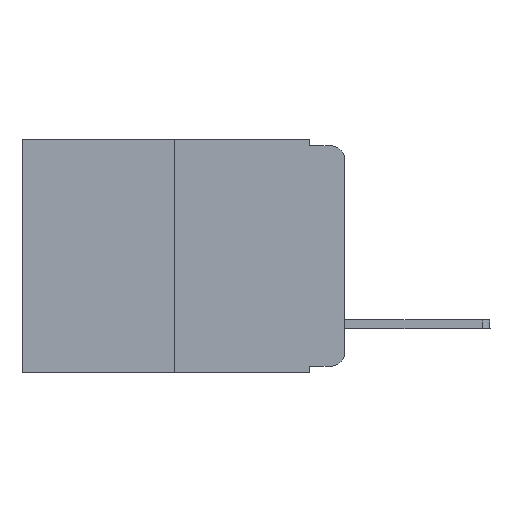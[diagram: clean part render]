
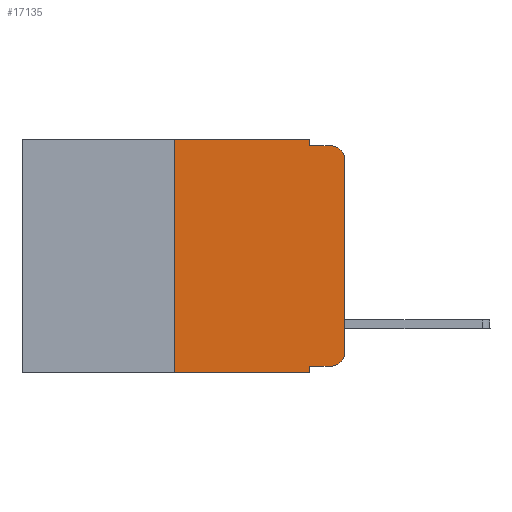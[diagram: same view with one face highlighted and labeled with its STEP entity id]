
A CAD part, left-side view. The second image highlights one B-rep face of the part: STEP entity #17135.
In plain terms, the highlighted planar face has unit normal (-1, 0, 0).
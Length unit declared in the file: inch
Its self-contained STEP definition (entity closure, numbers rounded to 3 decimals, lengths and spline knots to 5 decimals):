
#48 = VERTEX_POINT ( 'NONE', #3010 ) ;
#542 = DIRECTION ( 'NONE',  ( 0., -1., 0. ) ) ;
#660 = VERTEX_POINT ( 'NONE', #7264 ) ;
#1312 = LINE ( 'NONE', #23140, #12895 ) ;
#1496 = VERTEX_POINT ( 'NONE', #4946 ) ;
#1572 = FACE_OUTER_BOUND ( 'NONE', #9296, .T. ) ;
#1698 = CARTESIAN_POINT ( 'NONE',  ( 0., 0.02, -0.313 ) ) ;
#1851 = DIRECTION ( 'NONE',  ( 0., 0., 1. ) ) ;
#1903 = VERTEX_POINT ( 'NONE', #15312 ) ;
#2299 = AXIS2_PLACEMENT_3D ( 'NONE', #1698, #24420, #22490 ) ;
#2646 = CARTESIAN_POINT ( 'NONE',  ( 0., 0.051, -0.333 ) ) ;
#2754 = PLANE ( 'NONE',  #18215 ) ;
#2845 = EDGE_CURVE ( 'NONE', #12821, #1496, #10473, .T. ) ;
#3010 = CARTESIAN_POINT ( 'NONE',  ( 0., 0.25, -0.343 ) ) ;
#3219 = ORIENTED_EDGE ( 'NONE', *, *, #4584, .F. ) ;
#3416 = CARTESIAN_POINT ( 'NONE',  ( 0., 0., -0.03 ) ) ;
#3475 = EDGE_CURVE ( 'NONE', #10105, #660, #10136, .T. ) ;
#3656 = VERTEX_POINT ( 'NONE', #19422 ) ;
#4069 = ORIENTED_EDGE ( 'NONE', *, *, #13524, .T. ) ;
#4584 = EDGE_CURVE ( 'NONE', #48, #1903, #13107, .T. ) ;
#4709 = DIRECTION ( 'NONE',  ( 0., 0., -1. ) ) ;
#4946 = CARTESIAN_POINT ( 'NONE',  ( 0., 0.051, -0.343 ) ) ;
#5136 = CARTESIAN_POINT ( 'NONE',  ( 0., 0.25, 0. ) ) ;
#5215 = CARTESIAN_POINT ( 'NONE',  ( 0., 0.02, -0.333 ) ) ;
#5938 = ORIENTED_EDGE ( 'NONE', *, *, #7610, .T. ) ;
#7150 = VERTEX_POINT ( 'NONE', #14529 ) ;
#7264 = CARTESIAN_POINT ( 'NONE',  ( 0., 0.02, -0.01 ) ) ;
#7610 = EDGE_CURVE ( 'NONE', #12301, #3656, #8796, .T. ) ;
#8024 = VECTOR ( 'NONE', #16521, 39.37008 ) ;
#8070 = DIRECTION ( 'NONE',  ( 0., 0., -1. ) ) ;
#8228 = DIRECTION ( 'NONE',  ( 0., -1., 0. ) ) ;
#8554 = ORIENTED_EDGE ( 'NONE', *, *, #2845, .F. ) ;
#8601 = DIRECTION ( 'NONE',  ( 0., -1., 0. ) ) ;
#8715 = CARTESIAN_POINT ( 'NONE',  ( 0., 0.473, 0. ) ) ;
#8796 = CIRCLE ( 'NONE', #2299, 0.02 ) ;
#8934 = CARTESIAN_POINT ( 'NONE',  ( 0., 0.051, -0.01 ) ) ;
#8983 = CIRCLE ( 'NONE', #24585, 0.02 ) ;
#8996 = CARTESIAN_POINT ( 'NONE',  ( 0., 0., 0. ) ) ;
#9296 = EDGE_LOOP ( 'NONE', ( #17163, #12043, #20667, #19735, #17613, #3219, #17798, #8554, #4069, #5938 ) ) ;
#9581 = VECTOR ( 'NONE', #8601, 39.37008 ) ;
#10083 = CARTESIAN_POINT ( 'NONE',  ( 0., 0.02, -0.03 ) ) ;
#10105 = VERTEX_POINT ( 'NONE', #8934 ) ;
#10136 = LINE ( 'NONE', #15644, #19667 ) ;
#10473 = LINE ( 'NONE', #23336, #15208 ) ;
#10817 = CARTESIAN_POINT ( 'NONE',  ( 0., 0.051, 0. ) ) ;
#12043 = ORIENTED_EDGE ( 'NONE', *, *, #23755, .T. ) ;
#12059 = EDGE_CURVE ( 'NONE', #48, #1496, #1312, .T. ) ;
#12069 = DIRECTION ( 'NONE',  ( -1., 0., 0. ) ) ;
#12172 = DIRECTION ( 'NONE',  ( 0., 0., -1. ) ) ;
#12301 = VERTEX_POINT ( 'NONE', #5215 ) ;
#12720 = DIRECTION ( 'NONE',  ( 0., 0., -1. ) ) ;
#12821 = VERTEX_POINT ( 'NONE', #15557 ) ;
#12895 = VECTOR ( 'NONE', #8228, 39.37008 ) ;
#13107 = LINE ( 'NONE', #5136, #8024 ) ;
#13524 = EDGE_CURVE ( 'NONE', #12821, #12301, #19996, .T. ) ;
#14342 = VECTOR ( 'NONE', #1851, 39.37008 ) ;
#14529 = CARTESIAN_POINT ( 'NONE',  ( 0., 0.051, 0. ) ) ;
#15208 = VECTOR ( 'NONE', #12172, 39.37008 ) ;
#15312 = CARTESIAN_POINT ( 'NONE',  ( 0., 0.25, 0. ) ) ;
#15557 = CARTESIAN_POINT ( 'NONE',  ( 0., 0.051, -0.333 ) ) ;
#15644 = CARTESIAN_POINT ( 'NONE',  ( 0., 0.051, -0.01 ) ) ;
#16416 = CARTESIAN_POINT ( 'NONE',  ( 0., 0.473, 0. ) ) ;
#16521 = DIRECTION ( 'NONE',  ( 0., 0., 1. ) ) ;
#16718 = EDGE_CURVE ( 'NONE', #3656, #22264, #18551, .T. ) ;
#17135 = ADVANCED_FACE ( 'NONE', ( #1572 ), #2754, .F. ) ;
#17163 = ORIENTED_EDGE ( 'NONE', *, *, #16718, .T. ) ;
#17613 = ORIENTED_EDGE ( 'NONE', *, *, #17836, .F. ) ;
#17798 = ORIENTED_EDGE ( 'NONE', *, *, #12059, .T. ) ;
#17836 = EDGE_CURVE ( 'NONE', #1903, #7150, #19375, .T. ) ;
#18215 = AXIS2_PLACEMENT_3D ( 'NONE', #8715, #20111, #4709 ) ;
#18551 = LINE ( 'NONE', #8996, #14342 ) ;
#19375 = LINE ( 'NONE', #16416, #24165 ) ;
#19422 = CARTESIAN_POINT ( 'NONE',  ( 0., 0., -0.313 ) ) ;
#19667 = VECTOR ( 'NONE', #542, 39.37008 ) ;
#19735 = ORIENTED_EDGE ( 'NONE', *, *, #20704, .F. ) ;
#19996 = LINE ( 'NONE', #2646, #9581 ) ;
#20111 = DIRECTION ( 'NONE',  ( 1., 0., 0. ) ) ;
#20667 = ORIENTED_EDGE ( 'NONE', *, *, #3475, .F. ) ;
#20704 = EDGE_CURVE ( 'NONE', #7150, #10105, #21334, .T. ) ;
#21334 = LINE ( 'NONE', #10817, #23434 ) ;
#22183 = DIRECTION ( 'NONE',  ( 0., -1., 0. ) ) ;
#22264 = VERTEX_POINT ( 'NONE', #3416 ) ;
#22490 = DIRECTION ( 'NONE',  ( 0., 0., -1. ) ) ;
#23140 = CARTESIAN_POINT ( 'NONE',  ( 0., 0.473, -0.343 ) ) ;
#23336 = CARTESIAN_POINT ( 'NONE',  ( 0., 0.051, 0. ) ) ;
#23434 = VECTOR ( 'NONE', #12720, 39.37008 ) ;
#23755 = EDGE_CURVE ( 'NONE', #22264, #660, #8983, .T. ) ;
#24165 = VECTOR ( 'NONE', #22183, 39.37008 ) ;
#24420 = DIRECTION ( 'NONE',  ( -1., 0., 0. ) ) ;
#24585 = AXIS2_PLACEMENT_3D ( 'NONE', #10083, #12069, #8070 ) ;
